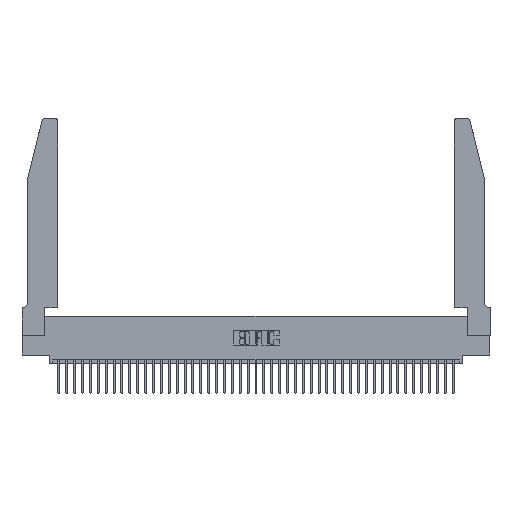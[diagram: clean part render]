
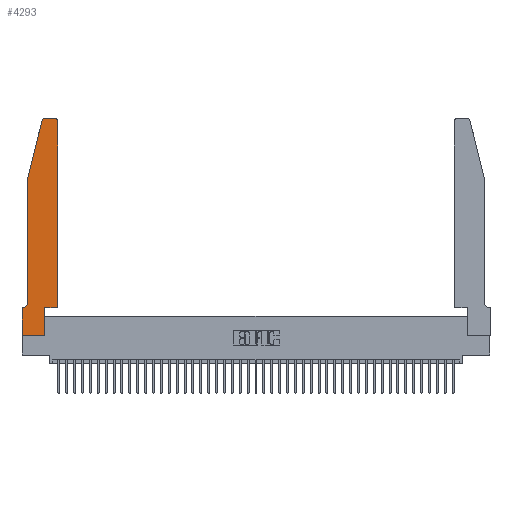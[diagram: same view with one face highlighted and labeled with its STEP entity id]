
A CAD part, top view. The second image highlights one B-rep face of the part: STEP entity #4293.
In plain terms, the highlighted planar face has unit normal (0, 0, 1).
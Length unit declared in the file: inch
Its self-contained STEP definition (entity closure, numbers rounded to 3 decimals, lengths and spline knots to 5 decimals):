
#465 = CARTESIAN_POINT ( 'NONE',  ( 0.0755, 2., 0.37 ) ) ;
#879 = EDGE_CURVE ( 'NONE', #13442, #11390, #19864, .T. ) ;
#1213 = CARTESIAN_POINT ( 'NONE',  ( 0., 0.35, 0.37 ) ) ;
#1887 = LINE ( 'NONE', #13306, #10923 ) ;
#2120 = CARTESIAN_POINT ( 'NONE',  ( 0.0055, 0.42, 0.37 ) ) ;
#2193 = VECTOR ( 'NONE', #14003, 39.37008 ) ;
#2355 = LINE ( 'NONE', #25043, #26222 ) ;
#2381 = DIRECTION ( 'NONE',  ( -1., 0., 0. ) ) ;
#3582 = ORIENTED_EDGE ( 'NONE', *, *, #879, .T. ) ;
#3610 = VECTOR ( 'NONE', #2381, 39.37008 ) ;
#4293 = ADVANCED_FACE ( 'NONE', ( #28496 ), #36575, .T. ) ;
#4639 = VERTEX_POINT ( 'NONE', #1213 ) ;
#4793 = CARTESIAN_POINT ( 'NONE',  ( 0.2865, 0., 0.37 ) ) ;
#4795 = CARTESIAN_POINT ( 'NONE',  ( 0.25487, 2.72718, 0.37 ) ) ;
#5551 = DIRECTION ( 'NONE',  ( -1., 0., 0. ) ) ;
#5769 = DIRECTION ( 'NONE',  ( 1., 0., 0. ) ) ;
#6327 = DIRECTION ( 'NONE',  ( 0., 0., 1. ) ) ;
#6487 = DIRECTION ( 'NONE',  ( 1., 0., 0. ) ) ;
#6592 = LINE ( 'NONE', #38477, #32463 ) ;
#6617 = CARTESIAN_POINT ( 'NONE',  ( 0.4505, 0.35, 0.37 ) ) ;
#6694 = VECTOR ( 'NONE', #37941, 39.37008 ) ;
#7670 = CIRCLE ( 'NONE', #42775, 0.07 ) ;
#7904 = CARTESIAN_POINT ( 'NONE',  ( 0.0755, 2., 0.37 ) ) ;
#9254 = VERTEX_POINT ( 'NONE', #4793 ) ;
#9968 = AXIS2_PLACEMENT_3D ( 'NONE', #35670, #15490, #39059 ) ;
#10923 = VECTOR ( 'NONE', #6487, 39.37008 ) ;
#11390 = VERTEX_POINT ( 'NONE', #23742 ) ;
#11491 = ORIENTED_EDGE ( 'NONE', *, *, #27898, .T. ) ;
#12595 = EDGE_CURVE ( 'NONE', #30101, #30284, #1887, .T. ) ;
#13306 = CARTESIAN_POINT ( 'NONE',  ( 0.4505, 0.35, 0.37 ) ) ;
#13442 = VERTEX_POINT ( 'NONE', #37175 ) ;
#13977 = VECTOR ( 'NONE', #19497, 39.37008 ) ;
#14003 = DIRECTION ( 'NONE',  ( 0., -1., 0. ) ) ;
#15328 = CARTESIAN_POINT ( 'NONE',  ( 0.4505, 0.35, 0.37 ) ) ;
#15490 = DIRECTION ( 'NONE',  ( 0., 0., 1. ) ) ;
#15701 = LINE ( 'NONE', #34547, #6694 ) ;
#15751 = ORIENTED_EDGE ( 'NONE', *, *, #16365, .T. ) ;
#15890 = CARTESIAN_POINT ( 'NONE',  ( 0.2605, 2.75, 0.37 ) ) ;
#16365 = EDGE_CURVE ( 'NONE', #29366, #9254, #6592, .T. ) ;
#16642 = EDGE_CURVE ( 'NONE', #9254, #30101, #39803, .T. ) ;
#17188 = CARTESIAN_POINT ( 'NONE',  ( 0., 0., 0.37 ) ) ;
#17229 = VERTEX_POINT ( 'NONE', #43519 ) ;
#17581 = VECTOR ( 'NONE', #40377, 39.37008 ) ;
#18101 = DIRECTION ( 'NONE',  ( -1., 0., 0. ) ) ;
#18640 = LINE ( 'NONE', #6617, #17581 ) ;
#19497 = DIRECTION ( 'NONE',  ( 0., 1., 0. ) ) ;
#19864 = CIRCLE ( 'NONE', #21759, 0.03 ) ;
#21038 = ORIENTED_EDGE ( 'NONE', *, *, #34681, .T. ) ;
#21085 = VERTEX_POINT ( 'NONE', #38263 ) ;
#21759 = AXIS2_PLACEMENT_3D ( 'NONE', #36325, #36276, #5769 ) ;
#22353 = LINE ( 'NONE', #465, #2193 ) ;
#23236 = EDGE_CURVE ( 'NONE', #30284, #13442, #18640, .T. ) ;
#23541 = CIRCLE ( 'NONE', #9968, 0.03 ) ;
#23742 = CARTESIAN_POINT ( 'NONE',  ( 0.4205, 2.75, 0.37 ) ) ;
#24232 = ORIENTED_EDGE ( 'NONE', *, *, #12595, .T. ) ;
#24500 = EDGE_LOOP ( 'NONE', ( #35182, #35732, #21038, #38901, #11491, #38399, #41522, #15751, #41011, #24232, #35262, #3582 ) ) ;
#25043 = CARTESIAN_POINT ( 'NONE',  ( 0.0755, 0.35, 0.37 ) ) ;
#25854 = DIRECTION ( 'NONE',  ( 0., 0., -1. ) ) ;
#26222 = VECTOR ( 'NONE', #18101, 39.37008 ) ;
#26623 = CARTESIAN_POINT ( 'NONE',  ( 0., 0.35, 0.37 ) ) ;
#27898 = EDGE_CURVE ( 'NONE', #17229, #21085, #7670, .T. ) ;
#28215 = VERTEX_POINT ( 'NONE', #4795 ) ;
#28350 = DIRECTION ( 'NONE',  ( 1., 0., 0. ) ) ;
#28496 = FACE_OUTER_BOUND ( 'NONE', #24500, .T. ) ;
#28909 = EDGE_CURVE ( 'NONE', #21085, #4639, #2355, .T. ) ;
#29013 = VECTOR ( 'NONE', #29746, 39.37008 ) ;
#29366 = VERTEX_POINT ( 'NONE', #17188 ) ;
#29746 = DIRECTION ( 'NONE',  ( 0., -1., 0. ) ) ;
#29968 = DIRECTION ( 'NONE',  ( 1., 0., 0. ) ) ;
#30101 = VERTEX_POINT ( 'NONE', #31245 ) ;
#30284 = VERTEX_POINT ( 'NONE', #15328 ) ;
#31245 = CARTESIAN_POINT ( 'NONE',  ( 0.2865, 0.35, 0.37 ) ) ;
#32463 = VECTOR ( 'NONE', #28350, 39.37008 ) ;
#34547 = CARTESIAN_POINT ( 'NONE',  ( 0.0755, 2., 0.37 ) ) ;
#34681 = EDGE_CURVE ( 'NONE', #28215, #37774, #15701, .T. ) ;
#35182 = ORIENTED_EDGE ( 'NONE', *, *, #43210, .T. ) ;
#35262 = ORIENTED_EDGE ( 'NONE', *, *, #23236, .T. ) ;
#35530 = EDGE_CURVE ( 'NONE', #40378, #28215, #23541, .T. ) ;
#35670 = CARTESIAN_POINT ( 'NONE',  ( 0.284, 2.72, 0.37 ) ) ;
#35732 = ORIENTED_EDGE ( 'NONE', *, *, #35530, .T. ) ;
#36276 = DIRECTION ( 'NONE',  ( 0., 0., 1. ) ) ;
#36325 = CARTESIAN_POINT ( 'NONE',  ( 0.4205, 2.72, 0.37 ) ) ;
#36364 = CARTESIAN_POINT ( 'NONE',  ( 0., 0., 0.37 ) ) ;
#36575 = PLANE ( 'NONE',  #43469 ) ;
#36745 = CARTESIAN_POINT ( 'NONE',  ( 0.284, 2.75, 0.37 ) ) ;
#37175 = CARTESIAN_POINT ( 'NONE',  ( 0.4505, 2.72, 0.37 ) ) ;
#37643 = EDGE_CURVE ( 'NONE', #37774, #17229, #22353, .T. ) ;
#37774 = VERTEX_POINT ( 'NONE', #7904 ) ;
#37919 = LINE ( 'NONE', #36364, #29013 ) ;
#37941 = DIRECTION ( 'NONE',  ( -0.239, -0.971, 0. ) ) ;
#38263 = CARTESIAN_POINT ( 'NONE',  ( 0.0055, 0.35, 0.37 ) ) ;
#38399 = ORIENTED_EDGE ( 'NONE', *, *, #28909, .T. ) ;
#38477 = CARTESIAN_POINT ( 'NONE',  ( 0., 0., 0.37 ) ) ;
#38901 = ORIENTED_EDGE ( 'NONE', *, *, #37643, .T. ) ;
#39059 = DIRECTION ( 'NONE',  ( 1., 0., 0. ) ) ;
#39525 = LINE ( 'NONE', #15890, #3610 ) ;
#39803 = LINE ( 'NONE', #43249, #13977 ) ;
#39934 = EDGE_CURVE ( 'NONE', #4639, #29366, #37919, .T. ) ;
#40377 = DIRECTION ( 'NONE',  ( 0., 1., 0. ) ) ;
#40378 = VERTEX_POINT ( 'NONE', #36745 ) ;
#41011 = ORIENTED_EDGE ( 'NONE', *, *, #16642, .T. ) ;
#41522 = ORIENTED_EDGE ( 'NONE', *, *, #39934, .T. ) ;
#42775 = AXIS2_PLACEMENT_3D ( 'NONE', #2120, #25854, #5551 ) ;
#43210 = EDGE_CURVE ( 'NONE', #11390, #40378, #39525, .T. ) ;
#43249 = CARTESIAN_POINT ( 'NONE',  ( 0.2865, 0.35, 0.37 ) ) ;
#43469 = AXIS2_PLACEMENT_3D ( 'NONE', #26623, #6327, #29968 ) ;
#43519 = CARTESIAN_POINT ( 'NONE',  ( 0.0755, 0.42, 0.37 ) ) ;
